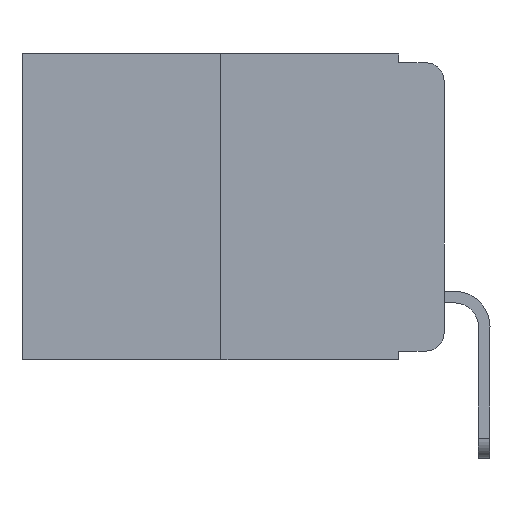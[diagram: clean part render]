
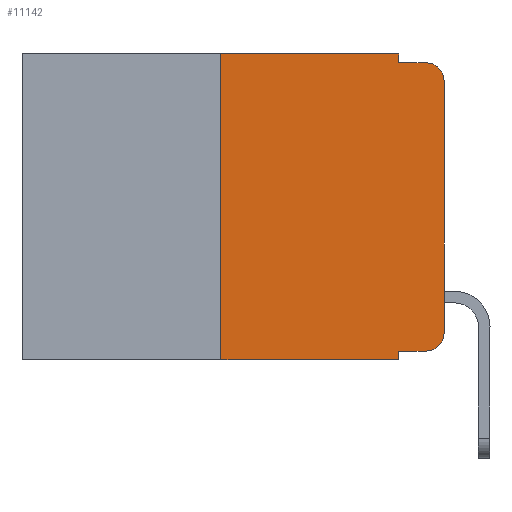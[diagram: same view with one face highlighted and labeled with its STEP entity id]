
A CAD part, left-side view. The second image highlights one B-rep face of the part: STEP entity #11142.
In plain terms, the highlighted planar face has unit normal (-1, 0, 0).
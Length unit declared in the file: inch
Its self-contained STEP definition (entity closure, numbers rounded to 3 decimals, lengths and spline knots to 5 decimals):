
#655 = DIRECTION ( 'NONE',  ( -1., 0., 0. ) ) ;
#1259 = VERTEX_POINT ( 'NONE', #10052 ) ;
#1295 = CARTESIAN_POINT ( 'NONE',  ( 0., 0.051, -0.01 ) ) ;
#1302 = VECTOR ( 'NONE', #16299, 39.37008 ) ;
#1342 = ORIENTED_EDGE ( 'NONE', *, *, #7186, .F. ) ;
#1494 = CARTESIAN_POINT ( 'NONE',  ( 0., 0.02, -0.333 ) ) ;
#2328 = ORIENTED_EDGE ( 'NONE', *, *, #8868, .F. ) ;
#2830 = LINE ( 'NONE', #8937, #7050 ) ;
#3101 = DIRECTION ( 'NONE',  ( 1., 0., 0. ) ) ;
#3188 = CARTESIAN_POINT ( 'NONE',  ( 0., 0.473, -0.343 ) ) ;
#3447 = EDGE_LOOP ( 'NONE', ( #15538, #4718, #12524, #2328, #3794, #1342, #5899, #16253, #14441, #14824 ) ) ;
#3534 = CIRCLE ( 'NONE', #16431, 0.02 ) ;
#3602 = DIRECTION ( 'NONE',  ( 0., -1., 0. ) ) ;
#3794 = ORIENTED_EDGE ( 'NONE', *, *, #9049, .F. ) ;
#3961 = VERTEX_POINT ( 'NONE', #7525 ) ;
#4354 = LINE ( 'NONE', #5886, #16847 ) ;
#4573 = AXIS2_PLACEMENT_3D ( 'NONE', #9637, #655, #12025 ) ;
#4718 = ORIENTED_EDGE ( 'NONE', *, *, #6798, .T. ) ;
#5286 = DIRECTION ( 'NONE',  ( -1., 0., 0. ) ) ;
#5397 = EDGE_CURVE ( 'NONE', #17537, #14127, #15887, .T. ) ;
#5886 = CARTESIAN_POINT ( 'NONE',  ( 0., 0., 0. ) ) ;
#5899 = ORIENTED_EDGE ( 'NONE', *, *, #15814, .T. ) ;
#6071 = CARTESIAN_POINT ( 'NONE',  ( 0., 0., -0.313 ) ) ;
#6460 = EDGE_CURVE ( 'NONE', #17537, #10583, #7122, .T. ) ;
#6798 = EDGE_CURVE ( 'NONE', #3961, #11496, #3534, .T. ) ;
#7050 = VECTOR ( 'NONE', #11664, 39.37008 ) ;
#7122 = LINE ( 'NONE', #16030, #15393 ) ;
#7186 = EDGE_CURVE ( 'NONE', #8822, #9369, #12911, .T. ) ;
#7393 = CARTESIAN_POINT ( 'NONE',  ( 0., 0.25, 0. ) ) ;
#7466 = DIRECTION ( 'NONE',  ( 0., -1., 0. ) ) ;
#7525 = CARTESIAN_POINT ( 'NONE',  ( 0., 0., -0.03 ) ) ;
#7893 = LINE ( 'NONE', #10688, #9472 ) ;
#8635 = CARTESIAN_POINT ( 'NONE',  ( 0., 0.25, 0. ) ) ;
#8822 = VERTEX_POINT ( 'NONE', #11725 ) ;
#8868 = EDGE_CURVE ( 'NONE', #1259, #18516, #2830, .T. ) ;
#8937 = CARTESIAN_POINT ( 'NONE',  ( 0., 0.051, 0. ) ) ;
#9049 = EDGE_CURVE ( 'NONE', #9369, #1259, #7893, .T. ) ;
#9369 = VERTEX_POINT ( 'NONE', #8635 ) ;
#9383 = VECTOR ( 'NONE', #18023, 39.37008 ) ;
#9472 = VECTOR ( 'NONE', #3602, 39.37008 ) ;
#9637 = CARTESIAN_POINT ( 'NONE',  ( 0., 0.02, -0.313 ) ) ;
#9793 = EDGE_CURVE ( 'NONE', #17677, #3961, #4354, .T. ) ;
#10052 = CARTESIAN_POINT ( 'NONE',  ( 0., 0.051, 0. ) ) ;
#10142 = AXIS2_PLACEMENT_3D ( 'NONE', #13895, #3101, #13075 ) ;
#10212 = LINE ( 'NONE', #10477, #1302 ) ;
#10477 = CARTESIAN_POINT ( 'NONE',  ( 0., 0.051, -0.01 ) ) ;
#10503 = DIRECTION ( 'NONE',  ( 0., 0., -1. ) ) ;
#10583 = VERTEX_POINT ( 'NONE', #13342 ) ;
#10684 = CARTESIAN_POINT ( 'NONE',  ( 0., 0.02, -0.01 ) ) ;
#10688 = CARTESIAN_POINT ( 'NONE',  ( 0., 0.473, 0. ) ) ;
#10873 = CARTESIAN_POINT ( 'NONE',  ( 0., 0.051, -0.333 ) ) ;
#11142 = ADVANCED_FACE ( 'NONE', ( #14553 ), #12301, .F. ) ;
#11493 = LINE ( 'NONE', #3188, #11708 ) ;
#11496 = VERTEX_POINT ( 'NONE', #10684 ) ;
#11664 = DIRECTION ( 'NONE',  ( 0., 0., -1. ) ) ;
#11708 = VECTOR ( 'NONE', #7466, 39.37008 ) ;
#11725 = CARTESIAN_POINT ( 'NONE',  ( 0., 0.25, -0.343 ) ) ;
#11740 = DIRECTION ( 'NONE',  ( 0., 0., 1. ) ) ;
#12025 = DIRECTION ( 'NONE',  ( 0., 0., -1. ) ) ;
#12301 = PLANE ( 'NONE',  #10142 ) ;
#12442 = CARTESIAN_POINT ( 'NONE',  ( 0., 0.02, -0.03 ) ) ;
#12524 = ORIENTED_EDGE ( 'NONE', *, *, #12947, .F. ) ;
#12911 = LINE ( 'NONE', #7393, #13333 ) ;
#12947 = EDGE_CURVE ( 'NONE', #18516, #11496, #10212, .T. ) ;
#13075 = DIRECTION ( 'NONE',  ( 0., 0., -1. ) ) ;
#13077 = CIRCLE ( 'NONE', #4573, 0.02 ) ;
#13333 = VECTOR ( 'NONE', #11740, 39.37008 ) ;
#13342 = CARTESIAN_POINT ( 'NONE',  ( 0., 0.051, -0.343 ) ) ;
#13895 = CARTESIAN_POINT ( 'NONE',  ( 0., 0.473, 0. ) ) ;
#14127 = VERTEX_POINT ( 'NONE', #1494 ) ;
#14310 = CARTESIAN_POINT ( 'NONE',  ( 0., 0.051, -0.333 ) ) ;
#14441 = ORIENTED_EDGE ( 'NONE', *, *, #5397, .T. ) ;
#14553 = FACE_OUTER_BOUND ( 'NONE', #3447, .T. ) ;
#14824 = ORIENTED_EDGE ( 'NONE', *, *, #14835, .T. ) ;
#14835 = EDGE_CURVE ( 'NONE', #14127, #17677, #13077, .T. ) ;
#15284 = DIRECTION ( 'NONE',  ( 0., 0., -1. ) ) ;
#15393 = VECTOR ( 'NONE', #10503, 39.37008 ) ;
#15538 = ORIENTED_EDGE ( 'NONE', *, *, #9793, .T. ) ;
#15814 = EDGE_CURVE ( 'NONE', #8822, #10583, #11493, .T. ) ;
#15878 = DIRECTION ( 'NONE',  ( 0., 0., 1. ) ) ;
#15887 = LINE ( 'NONE', #10873, #9383 ) ;
#16030 = CARTESIAN_POINT ( 'NONE',  ( 0., 0.051, 0. ) ) ;
#16253 = ORIENTED_EDGE ( 'NONE', *, *, #6460, .F. ) ;
#16299 = DIRECTION ( 'NONE',  ( 0., -1., 0. ) ) ;
#16431 = AXIS2_PLACEMENT_3D ( 'NONE', #12442, #5286, #15284 ) ;
#16847 = VECTOR ( 'NONE', #15878, 39.37008 ) ;
#17537 = VERTEX_POINT ( 'NONE', #14310 ) ;
#17677 = VERTEX_POINT ( 'NONE', #6071 ) ;
#18023 = DIRECTION ( 'NONE',  ( 0., -1., 0. ) ) ;
#18516 = VERTEX_POINT ( 'NONE', #1295 ) ;
